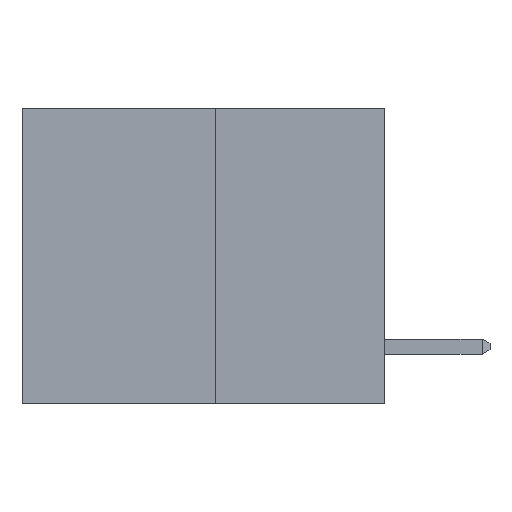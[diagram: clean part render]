
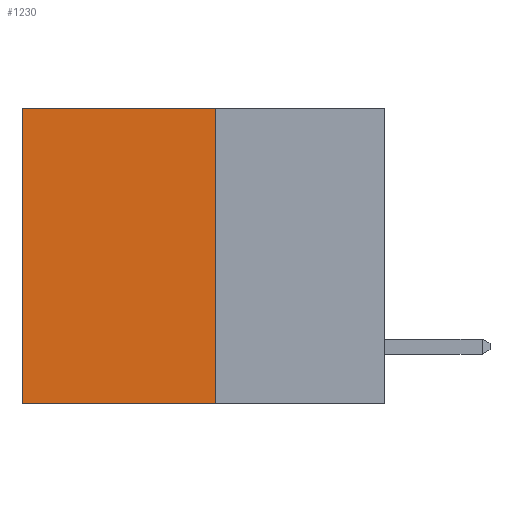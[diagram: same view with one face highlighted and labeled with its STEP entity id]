
A CAD part, left-side view. The second image highlights one B-rep face of the part: STEP entity #1230.
In plain terms, the highlighted planar face has unit normal (-1, 0, 0).
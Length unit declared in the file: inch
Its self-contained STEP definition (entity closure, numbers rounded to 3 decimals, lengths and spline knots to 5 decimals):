
#206 = ORIENTED_EDGE ( 'NONE', *, *, #7535, .F. ) ;
#418 = VECTOR ( 'NONE', #443, 39.37008 ) ;
#443 = DIRECTION ( 'NONE',  ( 0., 1., 0. ) ) ;
#655 = LINE ( 'NONE', #1971, #936 ) ;
#695 = DIRECTION ( 'NONE',  ( 0., 0., -1. ) ) ;
#917 = VECTOR ( 'NONE', #5162, 39.37008 ) ;
#936 = VECTOR ( 'NONE', #695, 39.37008 ) ;
#1057 = CARTESIAN_POINT ( 'NONE',  ( 0.3165, 0.6, 0. ) ) ;
#1230 = ADVANCED_FACE ( 'NONE', ( #5230 ), #4651, .F. ) ;
#1286 = CARTESIAN_POINT ( 'NONE',  ( 0.3165, 0.28, -0.49 ) ) ;
#1564 = DIRECTION ( 'NONE',  ( 0., 0., -1. ) ) ;
#1971 = CARTESIAN_POINT ( 'NONE',  ( 0.3165, 0.6, -0.49 ) ) ;
#2431 = ORIENTED_EDGE ( 'NONE', *, *, #7325, .F. ) ;
#2444 = AXIS2_PLACEMENT_3D ( 'NONE', #4031, #5206, #6488 ) ;
#2624 = LINE ( 'NONE', #5137, #917 ) ;
#3207 = VERTEX_POINT ( 'NONE', #1057 ) ;
#3869 = ORIENTED_EDGE ( 'NONE', *, *, #7745, .T. ) ;
#4031 = CARTESIAN_POINT ( 'NONE',  ( 0.3165, 0.28, -0.49 ) ) ;
#4379 = VERTEX_POINT ( 'NONE', #1286 ) ;
#4651 = PLANE ( 'NONE',  #2444 ) ;
#5137 = CARTESIAN_POINT ( 'NONE',  ( 0.3165, 0.28, -0.49 ) ) ;
#5162 = DIRECTION ( 'NONE',  ( 0., 1., 0. ) ) ;
#5206 = DIRECTION ( 'NONE',  ( 1., 0., 0. ) ) ;
#5230 = FACE_OUTER_BOUND ( 'NONE', #7921, .T. ) ;
#5536 = LINE ( 'NONE', #8218, #418 ) ;
#5777 = CARTESIAN_POINT ( 'NONE',  ( 0.3165, 0.28, 0. ) ) ;
#5796 = CARTESIAN_POINT ( 'NONE',  ( 0.3165, 0.6, -0.49 ) ) ;
#6039 = EDGE_CURVE ( 'NONE', #3207, #6832, #655, .T. ) ;
#6055 = VECTOR ( 'NONE', #1564, 39.37008 ) ;
#6464 = LINE ( 'NONE', #6726, #6055 ) ;
#6488 = DIRECTION ( 'NONE',  ( 0., 0., -1. ) ) ;
#6726 = CARTESIAN_POINT ( 'NONE',  ( 0.3165, 0.28, -0.49 ) ) ;
#6832 = VERTEX_POINT ( 'NONE', #5796 ) ;
#7325 = EDGE_CURVE ( 'NONE', #4379, #6832, #2624, .T. ) ;
#7535 = EDGE_CURVE ( 'NONE', #7830, #4379, #6464, .T. ) ;
#7745 = EDGE_CURVE ( 'NONE', #7830, #3207, #5536, .T. ) ;
#7830 = VERTEX_POINT ( 'NONE', #5777 ) ;
#7921 = EDGE_LOOP ( 'NONE', ( #8333, #2431, #206, #3869 ) ) ;
#8218 = CARTESIAN_POINT ( 'NONE',  ( 0.3165, 0.28, 0. ) ) ;
#8333 = ORIENTED_EDGE ( 'NONE', *, *, #6039, .T. ) ;
